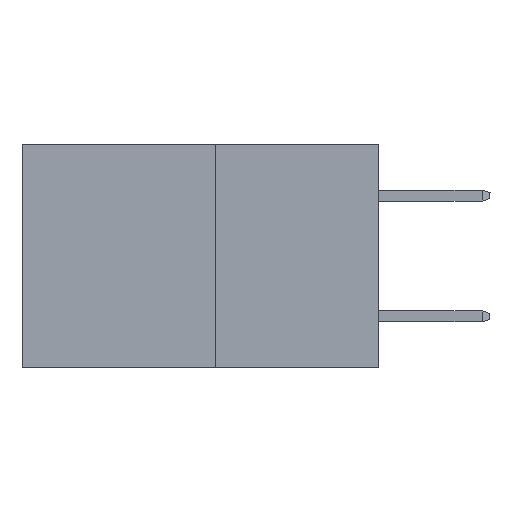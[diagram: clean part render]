
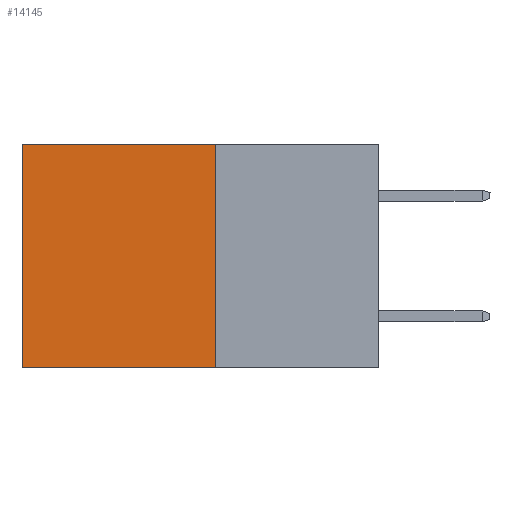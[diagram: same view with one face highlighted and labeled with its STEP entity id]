
A CAD part, left-side view. The second image highlights one B-rep face of the part: STEP entity #14145.
In plain terms, the highlighted planar face has unit normal (-1, 0, 0).
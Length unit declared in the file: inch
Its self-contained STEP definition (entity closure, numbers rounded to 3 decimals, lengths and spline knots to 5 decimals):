
#3 = DIRECTION ( 'NONE',  ( 1., 0., 0. ) ) ;
#83 = CARTESIAN_POINT ( 'NONE',  ( 0.277, 0.59, -0.37 ) ) ;
#249 = LINE ( 'NONE', #2239, #12462 ) ;
#342 = VERTEX_POINT ( 'NONE', #5684 ) ;
#923 = VERTEX_POINT ( 'NONE', #83 ) ;
#1210 = DIRECTION ( 'NONE',  ( 0., 1., 0. ) ) ;
#1596 = EDGE_CURVE ( 'NONE', #342, #11047, #9198, .T. ) ;
#2214 = CARTESIAN_POINT ( 'NONE',  ( 0.277, 0.27, 0. ) ) ;
#2239 = CARTESIAN_POINT ( 'NONE',  ( 0.277, 0.27, -0.37 ) ) ;
#2345 = ORIENTED_EDGE ( 'NONE', *, *, #15370, .F. ) ;
#2851 = CARTESIAN_POINT ( 'NONE',  ( 0.277, 0.27, -0.37 ) ) ;
#3102 = VECTOR ( 'NONE', #12697, 39.37008 ) ;
#3377 = AXIS2_PLACEMENT_3D ( 'NONE', #7357, #3, #8533 ) ;
#3764 = VECTOR ( 'NONE', #6198, 39.37008 ) ;
#3994 = ORIENTED_EDGE ( 'NONE', *, *, #5643, .F. ) ;
#5643 = EDGE_CURVE ( 'NONE', #14962, #923, #12875, .T. ) ;
#5684 = CARTESIAN_POINT ( 'NONE',  ( 0.277, 0.27, 0. ) ) ;
#5787 = ORIENTED_EDGE ( 'NONE', *, *, #1596, .T. ) ;
#6091 = PLANE ( 'NONE',  #3377 ) ;
#6198 = DIRECTION ( 'NONE',  ( 0., 0., -1. ) ) ;
#6307 = CARTESIAN_POINT ( 'NONE',  ( 0.277, 0.59, -0.37 ) ) ;
#7081 = LINE ( 'NONE', #6307, #3764 ) ;
#7357 = CARTESIAN_POINT ( 'NONE',  ( 0.277, 0.27, -0.37 ) ) ;
#8108 = CARTESIAN_POINT ( 'NONE',  ( 0.277, 0.59, 0. ) ) ;
#8533 = DIRECTION ( 'NONE',  ( 0., 0., -1. ) ) ;
#8812 = VECTOR ( 'NONE', #1210, 39.37008 ) ;
#9198 = LINE ( 'NONE', #2214, #8812 ) ;
#11047 = VERTEX_POINT ( 'NONE', #8108 ) ;
#11287 = EDGE_CURVE ( 'NONE', #11047, #923, #7081, .T. ) ;
#11724 = FACE_OUTER_BOUND ( 'NONE', #14457, .T. ) ;
#12028 = DIRECTION ( 'NONE',  ( 0., 0., -1. ) ) ;
#12462 = VECTOR ( 'NONE', #12028, 39.37008 ) ;
#12697 = DIRECTION ( 'NONE',  ( 0., 1., 0. ) ) ;
#12875 = LINE ( 'NONE', #2851, #3102 ) ;
#12997 = ORIENTED_EDGE ( 'NONE', *, *, #11287, .T. ) ;
#14145 = ADVANCED_FACE ( 'NONE', ( #11724 ), #6091, .F. ) ;
#14457 = EDGE_LOOP ( 'NONE', ( #12997, #3994, #2345, #5787 ) ) ;
#14962 = VERTEX_POINT ( 'NONE', #14998 ) ;
#14998 = CARTESIAN_POINT ( 'NONE',  ( 0.277, 0.27, -0.37 ) ) ;
#15370 = EDGE_CURVE ( 'NONE', #342, #14962, #249, .T. ) ;
